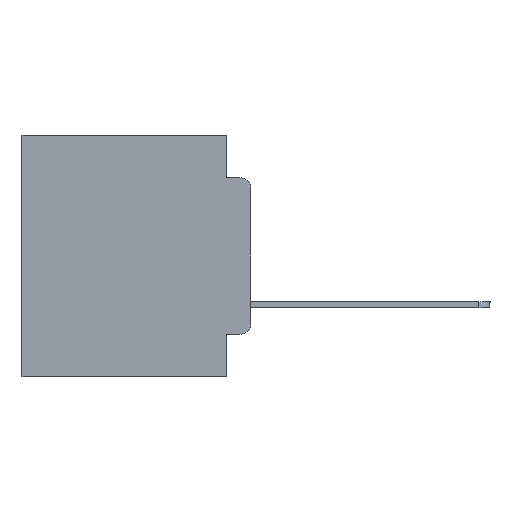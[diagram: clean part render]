
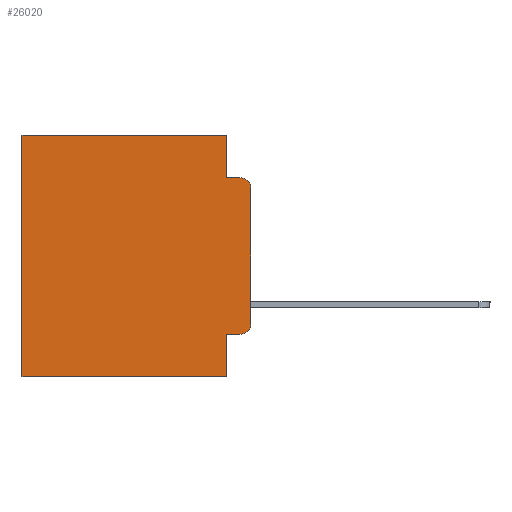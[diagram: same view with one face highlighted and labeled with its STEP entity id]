
A CAD part, left-side view. The second image highlights one B-rep face of the part: STEP entity #26020.
In plain terms, the highlighted planar face has unit normal (-1, 0, 0).
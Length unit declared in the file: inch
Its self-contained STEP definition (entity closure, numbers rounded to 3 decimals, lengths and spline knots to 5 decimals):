
#125 = DIRECTION ( 'NONE',  ( -1., 0., 0. ) ) ;
#180 = ORIENTED_EDGE ( 'NONE', *, *, #7787, .T. ) ;
#688 = VERTEX_POINT ( 'NONE', #9453 ) ;
#1015 = VECTOR ( 'NONE', #8418, 39.37008 ) ;
#1122 = LINE ( 'NONE', #14057, #8534 ) ;
#1204 = CARTESIAN_POINT ( 'NONE',  ( 0.298, 0.051, -0.4115 ) ) ;
#1351 = DIRECTION ( 'NONE',  ( 0., -1., 0. ) ) ;
#1486 = ORIENTED_EDGE ( 'NONE', *, *, #27503, .F. ) ;
#1487 = CIRCLE ( 'NONE', #21200, 0.02 ) ;
#1547 = VECTOR ( 'NONE', #19436, 39.37008 ) ;
#1645 = CIRCLE ( 'NONE', #13102, 0.02 ) ;
#1923 = LINE ( 'NONE', #10687, #1547 ) ;
#2056 = CARTESIAN_POINT ( 'NONE',  ( 0.298, 0., -0.5 ) ) ;
#2303 = ORIENTED_EDGE ( 'NONE', *, *, #5683, .F. ) ;
#2999 = DIRECTION ( 'NONE',  ( -1., 0., 0. ) ) ;
#3156 = EDGE_CURVE ( 'NONE', #9843, #16962, #1487, .T. ) ;
#3548 = ORIENTED_EDGE ( 'NONE', *, *, #12805, .F. ) ;
#3664 = CARTESIAN_POINT ( 'NONE',  ( 0.298, 0.051, 0. ) ) ;
#3751 = VERTEX_POINT ( 'NONE', #22794 ) ;
#4367 = DIRECTION ( 'NONE',  ( 0., 1., 0. ) ) ;
#4497 = VECTOR ( 'NONE', #7830, 39.37008 ) ;
#4659 = VERTEX_POINT ( 'NONE', #5905 ) ;
#4862 = VERTEX_POINT ( 'NONE', #18357 ) ;
#5683 = EDGE_CURVE ( 'NONE', #28070, #16962, #1923, .T. ) ;
#5905 = CARTESIAN_POINT ( 'NONE',  ( 0.298, 0.473, -0.5 ) ) ;
#6195 = FACE_OUTER_BOUND ( 'NONE', #26813, .T. ) ;
#6283 = CARTESIAN_POINT ( 'NONE',  ( 0.298, 0., 0. ) ) ;
#6523 = ORIENTED_EDGE ( 'NONE', *, *, #27778, .F. ) ;
#6990 = DIRECTION ( 'NONE',  ( 0., 0., -1. ) ) ;
#7389 = CARTESIAN_POINT ( 'NONE',  ( 0.298, 0., -0.1085 ) ) ;
#7787 = EDGE_CURVE ( 'NONE', #688, #19415, #1645, .T. ) ;
#7830 = DIRECTION ( 'NONE',  ( 0., 0., -1. ) ) ;
#7851 = EDGE_CURVE ( 'NONE', #4862, #4659, #1122, .T. ) ;
#8418 = DIRECTION ( 'NONE',  ( 0., 0., -1. ) ) ;
#8534 = VECTOR ( 'NONE', #12189, 39.37008 ) ;
#8711 = CARTESIAN_POINT ( 'NONE',  ( 0.298, 0.051, 0. ) ) ;
#8895 = DIRECTION ( 'NONE',  ( 0., 0., -1. ) ) ;
#9448 = AXIS2_PLACEMENT_3D ( 'NONE', #10507, #23696, #12652 ) ;
#9453 = CARTESIAN_POINT ( 'NONE',  ( 0.298, 0.02, -0.4115 ) ) ;
#9678 = CARTESIAN_POINT ( 'NONE',  ( 0.298, 0.051, -0.0885 ) ) ;
#9843 = VERTEX_POINT ( 'NONE', #7389 ) ;
#9993 = LINE ( 'NONE', #3664, #4497 ) ;
#10507 = CARTESIAN_POINT ( 'NONE',  ( 0.298, 0., 0. ) ) ;
#10531 = ORIENTED_EDGE ( 'NONE', *, *, #3156, .T. ) ;
#10687 = CARTESIAN_POINT ( 'NONE',  ( 0.298, 0.051, -0.0885 ) ) ;
#12189 = DIRECTION ( 'NONE',  ( 0., 0., -1. ) ) ;
#12652 = DIRECTION ( 'NONE',  ( 0., 0., -1. ) ) ;
#12777 = VECTOR ( 'NONE', #1351, 39.37008 ) ;
#12805 = EDGE_CURVE ( 'NONE', #24507, #4659, #17004, .T. ) ;
#13102 = AXIS2_PLACEMENT_3D ( 'NONE', #20652, #2999, #24961 ) ;
#13631 = CARTESIAN_POINT ( 'NONE',  ( 0.298, 0.02, -0.1085 ) ) ;
#14057 = CARTESIAN_POINT ( 'NONE',  ( 0.298, 0.473, 0. ) ) ;
#14566 = VERTEX_POINT ( 'NONE', #24576 ) ;
#14644 = VECTOR ( 'NONE', #4367, 39.37008 ) ;
#15985 = CARTESIAN_POINT ( 'NONE',  ( 0.298, 0.051, -0.5 ) ) ;
#16223 = ORIENTED_EDGE ( 'NONE', *, *, #24203, .T. ) ;
#16296 = ORIENTED_EDGE ( 'NONE', *, *, #23046, .T. ) ;
#16407 = EDGE_CURVE ( 'NONE', #9843, #19415, #19608, .T. ) ;
#16714 = ORIENTED_EDGE ( 'NONE', *, *, #7851, .T. ) ;
#16962 = VERTEX_POINT ( 'NONE', #22414 ) ;
#17004 = LINE ( 'NONE', #2056, #14644 ) ;
#17041 = LINE ( 'NONE', #6283, #19585 ) ;
#18357 = CARTESIAN_POINT ( 'NONE',  ( 0.298, 0.473, 0. ) ) ;
#18377 = ORIENTED_EDGE ( 'NONE', *, *, #16407, .F. ) ;
#18901 = DIRECTION ( 'NONE',  ( 0., 1., 0. ) ) ;
#19415 = VERTEX_POINT ( 'NONE', #27915 ) ;
#19436 = DIRECTION ( 'NONE',  ( 0., -1., 0. ) ) ;
#19585 = VECTOR ( 'NONE', #18901, 39.37008 ) ;
#19608 = LINE ( 'NONE', #25926, #1015 ) ;
#20069 = VECTOR ( 'NONE', #6990, 39.37008 ) ;
#20652 = CARTESIAN_POINT ( 'NONE',  ( 0.298, 0.02, -0.3915 ) ) ;
#20874 = LINE ( 'NONE', #1204, #12777 ) ;
#21200 = AXIS2_PLACEMENT_3D ( 'NONE', #13631, #125, #8895 ) ;
#22039 = LINE ( 'NONE', #8711, #20069 ) ;
#22414 = CARTESIAN_POINT ( 'NONE',  ( 0.298, 0.02, -0.0885 ) ) ;
#22794 = CARTESIAN_POINT ( 'NONE',  ( 0.298, 0.051, -0.4115 ) ) ;
#23046 = EDGE_CURVE ( 'NONE', #14566, #4862, #17041, .T. ) ;
#23696 = DIRECTION ( 'NONE',  ( 1., 0., 0. ) ) ;
#23839 = PLANE ( 'NONE',  #9448 ) ;
#24203 = EDGE_CURVE ( 'NONE', #3751, #688, #20874, .T. ) ;
#24507 = VERTEX_POINT ( 'NONE', #15985 ) ;
#24576 = CARTESIAN_POINT ( 'NONE',  ( 0.298, 0.051, 0. ) ) ;
#24961 = DIRECTION ( 'NONE',  ( 0., 0., -1. ) ) ;
#25926 = CARTESIAN_POINT ( 'NONE',  ( 0.298, 0., 0. ) ) ;
#26020 = ADVANCED_FACE ( 'NONE', ( #6195 ), #23839, .F. ) ;
#26813 = EDGE_LOOP ( 'NONE', ( #18377, #10531, #2303, #6523, #16296, #16714, #3548, #1486, #16223, #180 ) ) ;
#27503 = EDGE_CURVE ( 'NONE', #3751, #24507, #22039, .T. ) ;
#27778 = EDGE_CURVE ( 'NONE', #14566, #28070, #9993, .T. ) ;
#27915 = CARTESIAN_POINT ( 'NONE',  ( 0.298, 0., -0.3915 ) ) ;
#28070 = VERTEX_POINT ( 'NONE', #9678 ) ;
